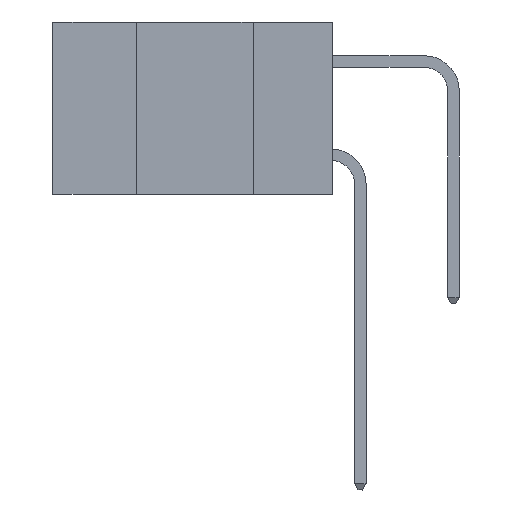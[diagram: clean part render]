
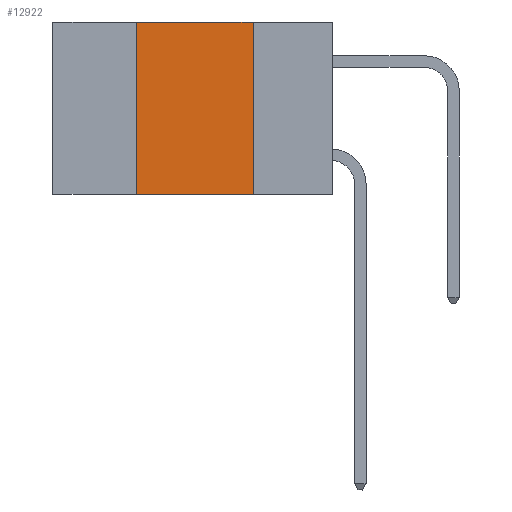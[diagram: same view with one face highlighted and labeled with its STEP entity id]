
A CAD part, left-side view. The second image highlights one B-rep face of the part: STEP entity #12922.
In plain terms, the highlighted planar face has unit normal (-1, 0, 0).
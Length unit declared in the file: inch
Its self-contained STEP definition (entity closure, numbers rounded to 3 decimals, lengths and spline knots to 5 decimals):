
#111 = VECTOR ( 'NONE', #13461, 39.37008 ) ;
#236 = VERTEX_POINT ( 'NONE', #24853 ) ;
#349 = ORIENTED_EDGE ( 'NONE', *, *, #27064, .F. ) ;
#3148 = LINE ( 'NONE', #13774, #21632 ) ;
#3593 = CARTESIAN_POINT ( 'NONE',  ( 0., 0.6, 0. ) ) ;
#3699 = VERTEX_POINT ( 'NONE', #15388 ) ;
#4876 = EDGE_LOOP ( 'NONE', ( #349, #15896, #26940, #22727 ) ) ;
#5645 = DIRECTION ( 'NONE',  ( 0., 0., -1. ) ) ;
#7289 = DIRECTION ( 'NONE',  ( 0., 0., 1. ) ) ;
#7902 = DIRECTION ( 'NONE',  ( 1., 0., 0. ) ) ;
#10015 = CARTESIAN_POINT ( 'NONE',  ( 0., 0.42, -0.37 ) ) ;
#11124 = EDGE_CURVE ( 'NONE', #236, #29709, #23224, .T. ) ;
#12340 = VECTOR ( 'NONE', #29916, 39.37008 ) ;
#12770 = EDGE_CURVE ( 'NONE', #25717, #236, #3148, .T. ) ;
#12922 = ADVANCED_FACE ( 'NONE', ( #24506 ), #15071, .F. ) ;
#13461 = DIRECTION ( 'NONE',  ( 0., -1., 0. ) ) ;
#13774 = CARTESIAN_POINT ( 'NONE',  ( 0., 0.42, 0. ) ) ;
#14686 = EDGE_CURVE ( 'NONE', #25717, #3699, #29445, .T. ) ;
#15071 = PLANE ( 'NONE',  #21294 ) ;
#15388 = CARTESIAN_POINT ( 'NONE',  ( 0., 0.17, -0.37 ) ) ;
#15896 = ORIENTED_EDGE ( 'NONE', *, *, #11124, .F. ) ;
#18039 = VECTOR ( 'NONE', #24092, 39.37008 ) ;
#21294 = AXIS2_PLACEMENT_3D ( 'NONE', #3593, #7902, #5645 ) ;
#21348 = CARTESIAN_POINT ( 'NONE',  ( 0., 0.17, 0. ) ) ;
#21632 = VECTOR ( 'NONE', #7289, 39.37008 ) ;
#21639 = LINE ( 'NONE', #23877, #18039 ) ;
#22727 = ORIENTED_EDGE ( 'NONE', *, *, #14686, .T. ) ;
#22786 = CARTESIAN_POINT ( 'NONE',  ( 0., 0.6, -0.37 ) ) ;
#23224 = LINE ( 'NONE', #26955, #12340 ) ;
#23877 = CARTESIAN_POINT ( 'NONE',  ( 0., 0.17, 0. ) ) ;
#24092 = DIRECTION ( 'NONE',  ( 0., 0., -1. ) ) ;
#24506 = FACE_OUTER_BOUND ( 'NONE', #4876, .T. ) ;
#24853 = CARTESIAN_POINT ( 'NONE',  ( 0., 0.42, 0. ) ) ;
#25717 = VERTEX_POINT ( 'NONE', #10015 ) ;
#26940 = ORIENTED_EDGE ( 'NONE', *, *, #12770, .F. ) ;
#26955 = CARTESIAN_POINT ( 'NONE',  ( 0., 0.6, 0. ) ) ;
#27064 = EDGE_CURVE ( 'NONE', #29709, #3699, #21639, .T. ) ;
#29445 = LINE ( 'NONE', #22786, #111 ) ;
#29709 = VERTEX_POINT ( 'NONE', #21348 ) ;
#29916 = DIRECTION ( 'NONE',  ( 0., -1., 0. ) ) ;
